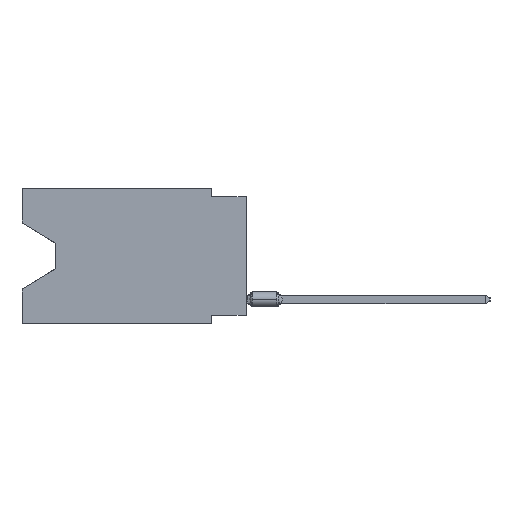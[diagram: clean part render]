
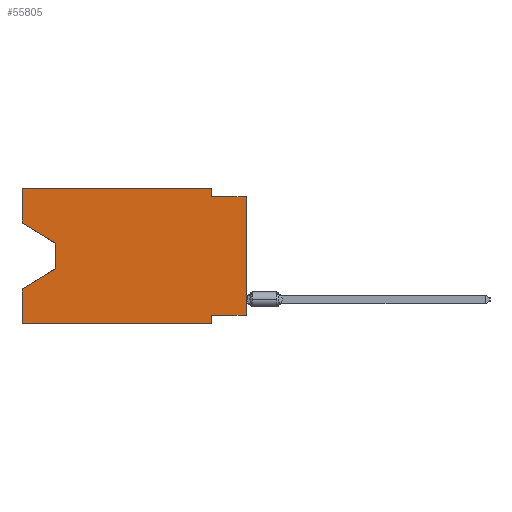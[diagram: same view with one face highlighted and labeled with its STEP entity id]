
A CAD part, left-side view. The second image highlights one B-rep face of the part: STEP entity #55805.
In plain terms, the highlighted planar face has unit normal (-1, 0, 0).
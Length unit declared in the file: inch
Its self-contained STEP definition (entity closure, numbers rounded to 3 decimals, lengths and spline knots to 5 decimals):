
#72 = DIRECTION ( 'NONE',  ( 0., -1., 0. ) ) ;
#1547 = EDGE_CURVE ( 'NONE', #26220, #30597, #17835, .T. ) ;
#1825 = CARTESIAN_POINT ( 'NONE',  ( 0., 0., -0.365 ) ) ;
#2050 = LINE ( 'NONE', #28160, #17615 ) ;
#3026 = CARTESIAN_POINT ( 'NONE',  ( 0., 0.645, 0. ) ) ;
#3443 = CARTESIAN_POINT ( 'NONE',  ( 0., 0.1, -0.39 ) ) ;
#3493 = CARTESIAN_POINT ( 'NONE',  ( 0., 0.645, -0.10025 ) ) ;
#3859 = CARTESIAN_POINT ( 'NONE',  ( 0., 0.645, 0. ) ) ;
#6167 = ORIENTED_EDGE ( 'NONE', *, *, #25154, .F. ) ;
#6640 = DIRECTION ( 'NONE',  ( 0., 0., 1. ) ) ;
#6878 = PLANE ( 'NONE',  #53377 ) ;
#7283 = VECTOR ( 'NONE', #29102, 39.37008 ) ;
#7527 = DIRECTION ( 'NONE',  ( 0., 0.855, -0.519 ) ) ;
#8398 = VECTOR ( 'NONE', #6640, 39.37008 ) ;
#8628 = LINE ( 'NONE', #44661, #49619 ) ;
#8657 = ORIENTED_EDGE ( 'NONE', *, *, #51102, .F. ) ;
#9451 = LINE ( 'NONE', #27319, #12415 ) ;
#9682 = ORIENTED_EDGE ( 'NONE', *, *, #34557, .F. ) ;
#9905 = ORIENTED_EDGE ( 'NONE', *, *, #25322, .F. ) ;
#10215 = VECTOR ( 'NONE', #7527, 39.37008 ) ;
#10301 = EDGE_CURVE ( 'NONE', #40926, #10732, #16739, .T. ) ;
#10732 = VERTEX_POINT ( 'NONE', #31825 ) ;
#10795 = CARTESIAN_POINT ( 'NONE',  ( 0., 0., -0.365 ) ) ;
#11186 = ORIENTED_EDGE ( 'NONE', *, *, #37906, .F. ) ;
#11248 = LINE ( 'NONE', #1825, #7283 ) ;
#11596 = ORIENTED_EDGE ( 'NONE', *, *, #55262, .T. ) ;
#11706 = VECTOR ( 'NONE', #53599, 39.37008 ) ;
#11711 = ORIENTED_EDGE ( 'NONE', *, *, #40714, .T. ) ;
#12415 = VECTOR ( 'NONE', #45202, 39.37008 ) ;
#15799 = EDGE_CURVE ( 'NONE', #40926, #43140, #2050, .T. ) ;
#16553 = CARTESIAN_POINT ( 'NONE',  ( 0., 0.1, 0. ) ) ;
#16739 = LINE ( 'NONE', #3493, #51066 ) ;
#17615 = VECTOR ( 'NONE', #19969, 39.37008 ) ;
#17835 = LINE ( 'NONE', #35702, #11706 ) ;
#19409 = CARTESIAN_POINT ( 'NONE',  ( 0., 0., -0.025 ) ) ;
#19549 = CARTESIAN_POINT ( 'NONE',  ( 0., 0., 0. ) ) ;
#19969 = DIRECTION ( 'NONE',  ( 0., 0., 1. ) ) ;
#20108 = CARTESIAN_POINT ( 'NONE',  ( 0., 0.55, -0.232 ) ) ;
#20833 = DIRECTION ( 'NONE',  ( 0., -0.855, -0.519 ) ) ;
#21225 = FACE_OUTER_BOUND ( 'NONE', #43575, .T. ) ;
#21328 = DIRECTION ( 'NONE',  ( 0., 0., -1. ) ) ;
#21478 = DIRECTION ( 'NONE',  ( 0., -1., 0. ) ) ;
#22011 = VERTEX_POINT ( 'NONE', #27826 ) ;
#22067 = DIRECTION ( 'NONE',  ( 0., 0., -1. ) ) ;
#22110 = ORIENTED_EDGE ( 'NONE', *, *, #10301, .T. ) ;
#22494 = CARTESIAN_POINT ( 'NONE',  ( 0., 0.645, 0. ) ) ;
#23264 = VECTOR ( 'NONE', #22067, 39.37008 ) ;
#23359 = LINE ( 'NONE', #19549, #8398 ) ;
#23908 = CARTESIAN_POINT ( 'NONE',  ( 0., 0.645, -0.10025 ) ) ;
#25154 = EDGE_CURVE ( 'NONE', #43140, #34921, #53428, .T. ) ;
#25322 = EDGE_CURVE ( 'NONE', #27968, #26390, #9451, .T. ) ;
#25401 = CARTESIAN_POINT ( 'NONE',  ( 0., 0.55, -0.232 ) ) ;
#26220 = VERTEX_POINT ( 'NONE', #47611 ) ;
#26390 = VERTEX_POINT ( 'NONE', #19409 ) ;
#27319 = CARTESIAN_POINT ( 'NONE',  ( 0., 0., -0.025 ) ) ;
#27826 = CARTESIAN_POINT ( 'NONE',  ( 0., 0.645, -0.39 ) ) ;
#27912 = VERTEX_POINT ( 'NONE', #10795 ) ;
#27968 = VERTEX_POINT ( 'NONE', #42434 ) ;
#28160 = CARTESIAN_POINT ( 'NONE',  ( 0., 0.645, 0. ) ) ;
#29102 = DIRECTION ( 'NONE',  ( 0., 1., 0. ) ) ;
#29442 = VERTEX_POINT ( 'NONE', #56833 ) ;
#30044 = ORIENTED_EDGE ( 'NONE', *, *, #35230, .T. ) ;
#30597 = VERTEX_POINT ( 'NONE', #3443 ) ;
#30842 = VECTOR ( 'NONE', #45680, 39.37008 ) ;
#31825 = CARTESIAN_POINT ( 'NONE',  ( 0., 0.55, -0.158 ) ) ;
#32483 = ORIENTED_EDGE ( 'NONE', *, *, #1547, .F. ) ;
#33813 = DIRECTION ( 'NONE',  ( 1., 0., 0. ) ) ;
#34557 = EDGE_CURVE ( 'NONE', #34921, #27968, #34679, .T. ) ;
#34679 = LINE ( 'NONE', #16553, #23264 ) ;
#34921 = VERTEX_POINT ( 'NONE', #35679 ) ;
#35230 = EDGE_CURVE ( 'NONE', #50646, #29442, #42966, .T. ) ;
#35679 = CARTESIAN_POINT ( 'NONE',  ( 0., 0.1, 0. ) ) ;
#35702 = CARTESIAN_POINT ( 'NONE',  ( 0., 0.1, -0.39 ) ) ;
#35900 = EDGE_CURVE ( 'NONE', #22011, #30597, #8628, .T. ) ;
#37906 = EDGE_CURVE ( 'NONE', #22011, #29442, #54494, .T. ) ;
#40714 = EDGE_CURVE ( 'NONE', #10732, #50646, #43876, .T. ) ;
#40926 = VERTEX_POINT ( 'NONE', #23908 ) ;
#42434 = CARTESIAN_POINT ( 'NONE',  ( 0., 0.1, -0.025 ) ) ;
#42966 = LINE ( 'NONE', #25401, #10215 ) ;
#43140 = VERTEX_POINT ( 'NONE', #22494 ) ;
#43575 = EDGE_LOOP ( 'NONE', ( #22110, #11711, #30044, #11186, #46086, #32483, #8657, #11596, #9905, #9682, #6167, #46282 ) ) ;
#43595 = CARTESIAN_POINT ( 'NONE',  ( 0., 0.55, -0.158 ) ) ;
#43876 = LINE ( 'NONE', #43595, #46061 ) ;
#44661 = CARTESIAN_POINT ( 'NONE',  ( 0., 0.645, -0.39 ) ) ;
#45202 = DIRECTION ( 'NONE',  ( 0., -1., 0. ) ) ;
#45680 = DIRECTION ( 'NONE',  ( 0., 0., 1. ) ) ;
#45964 = CARTESIAN_POINT ( 'NONE',  ( 0., 0.645, 0. ) ) ;
#46061 = VECTOR ( 'NONE', #21328, 39.37008 ) ;
#46086 = ORIENTED_EDGE ( 'NONE', *, *, #35900, .T. ) ;
#46282 = ORIENTED_EDGE ( 'NONE', *, *, #15799, .F. ) ;
#47611 = CARTESIAN_POINT ( 'NONE',  ( 0., 0.1, -0.365 ) ) ;
#49619 = VECTOR ( 'NONE', #72, 39.37008 ) ;
#50646 = VERTEX_POINT ( 'NONE', #20108 ) ;
#51066 = VECTOR ( 'NONE', #20833, 39.37008 ) ;
#51102 = EDGE_CURVE ( 'NONE', #27912, #26220, #11248, .T. ) ;
#51739 = VECTOR ( 'NONE', #21478, 39.37008 ) ;
#52590 = DIRECTION ( 'NONE',  ( 0., 0., -1. ) ) ;
#53377 = AXIS2_PLACEMENT_3D ( 'NONE', #3026, #33813, #52590 ) ;
#53428 = LINE ( 'NONE', #3859, #51739 ) ;
#53599 = DIRECTION ( 'NONE',  ( 0., 0., -1. ) ) ;
#54494 = LINE ( 'NONE', #45964, #30842 ) ;
#55262 = EDGE_CURVE ( 'NONE', #27912, #26390, #23359, .T. ) ;
#55805 = ADVANCED_FACE ( 'NONE', ( #21225 ), #6878, .F. ) ;
#56833 = CARTESIAN_POINT ( 'NONE',  ( 0., 0.645, -0.28975 ) ) ;
